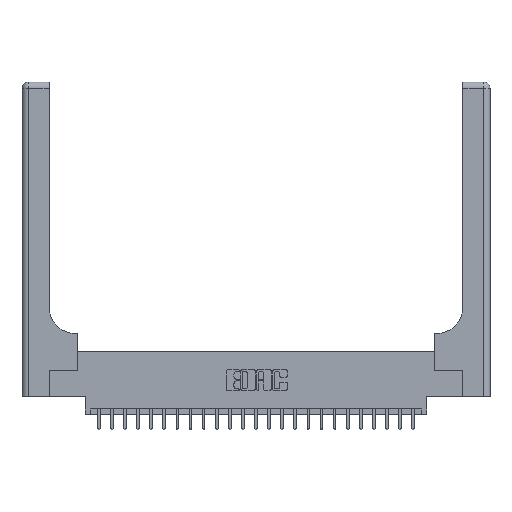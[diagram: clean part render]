
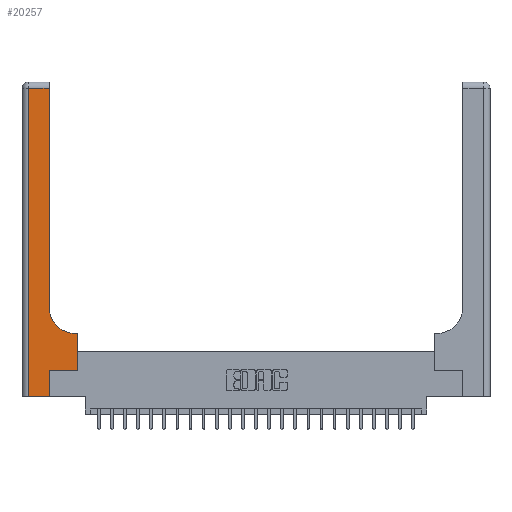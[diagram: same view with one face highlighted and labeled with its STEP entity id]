
A CAD part, top view. The second image highlights one B-rep face of the part: STEP entity #20257.
In plain terms, the highlighted planar face has unit normal (0, 0, 1).
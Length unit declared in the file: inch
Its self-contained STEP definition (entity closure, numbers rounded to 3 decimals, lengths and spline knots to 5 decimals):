
#1198 = CARTESIAN_POINT ( 'NONE',  ( 0.06, 3., 0.37 ) ) ;
#1529 = ORIENTED_EDGE ( 'NONE', *, *, #15188, .T. ) ;
#1655 = EDGE_CURVE ( 'NONE', #21835, #8231, #21204, .T. ) ;
#2003 = ORIENTED_EDGE ( 'NONE', *, *, #1655, .T. ) ;
#2154 = DIRECTION ( 'NONE',  ( 0., 1., 0. ) ) ;
#2416 = CARTESIAN_POINT ( 'NONE',  ( 0.26, 0.6, 0.37 ) ) ;
#2769 = ORIENTED_EDGE ( 'NONE', *, *, #5787, .T. ) ;
#2866 = DIRECTION ( 'NONE',  ( 1., 0., 0. ) ) ;
#3579 = DIRECTION ( 'NONE',  ( -1., 0., 0. ) ) ;
#4406 = DIRECTION ( 'NONE',  ( -1., 0., 0. ) ) ;
#4683 = DIRECTION ( 'NONE',  ( 0., 1., 0. ) ) ;
#4756 = LINE ( 'NONE', #6605, #23250 ) ;
#5188 = EDGE_CURVE ( 'NONE', #18639, #13208, #23554, .T. ) ;
#5787 = EDGE_CURVE ( 'NONE', #13319, #10318, #20450, .T. ) ;
#5858 = VERTEX_POINT ( 'NONE', #20570 ) ;
#6161 = LINE ( 'NONE', #14044, #10819 ) ;
#6267 = CARTESIAN_POINT ( 'NONE',  ( 0., 3., 0.37 ) ) ;
#6526 = ORIENTED_EDGE ( 'NONE', *, *, #8241, .T. ) ;
#6605 = CARTESIAN_POINT ( 'NONE',  ( 0.265, 0.25, 0.37 ) ) ;
#6738 = EDGE_CURVE ( 'NONE', #8231, #14518, #20949, .T. ) ;
#8231 = VERTEX_POINT ( 'NONE', #15338 ) ;
#8241 = EDGE_CURVE ( 'NONE', #13208, #13319, #6161, .T. ) ;
#8247 = DIRECTION ( 'NONE',  ( 1., 0., 0. ) ) ;
#8260 = EDGE_CURVE ( 'NONE', #5858, #18092, #11846, .T. ) ;
#8460 = VECTOR ( 'NONE', #4683, 39.37008 ) ;
#9105 = CARTESIAN_POINT ( 'NONE',  ( 0.06, 0., 0.37 ) ) ;
#9468 = CARTESIAN_POINT ( 'NONE',  ( 0.51, 0.6, 0.37 ) ) ;
#9710 = CARTESIAN_POINT ( 'NONE',  ( 0.265, 0., 0.37 ) ) ;
#9913 = EDGE_CURVE ( 'NONE', #18092, #21835, #10314, .T. ) ;
#10186 = AXIS2_PLACEMENT_3D ( 'NONE', #6267, #23171, #13796 ) ;
#10314 = LINE ( 'NONE', #2416, #19960 ) ;
#10318 = VERTEX_POINT ( 'NONE', #14209 ) ;
#10442 = VECTOR ( 'NONE', #3579, 39.37008 ) ;
#10819 = VECTOR ( 'NONE', #8247, 39.37008 ) ;
#11393 = VECTOR ( 'NONE', #19492, 39.37008 ) ;
#11846 = LINE ( 'NONE', #15560, #8460 ) ;
#13176 = CARTESIAN_POINT ( 'NONE',  ( 0.265, 0., 0.37 ) ) ;
#13208 = VERTEX_POINT ( 'NONE', #9105 ) ;
#13319 = VERTEX_POINT ( 'NONE', #9710 ) ;
#13342 = ORIENTED_EDGE ( 'NONE', *, *, #9913, .T. ) ;
#13569 = FACE_OUTER_BOUND ( 'NONE', #17978, .T. ) ;
#13658 = CARTESIAN_POINT ( 'NONE',  ( 0.26, 3., 0.37 ) ) ;
#13796 = DIRECTION ( 'NONE',  ( -1., 0., 0. ) ) ;
#14016 = CARTESIAN_POINT ( 'NONE',  ( 0.528, 0.6, 0.37 ) ) ;
#14044 = CARTESIAN_POINT ( 'NONE',  ( 0., 0., 0.37 ) ) ;
#14209 = CARTESIAN_POINT ( 'NONE',  ( 0.265, 0.25, 0.37 ) ) ;
#14497 = CARTESIAN_POINT ( 'NONE',  ( 0.06, 2.94, 0.37 ) ) ;
#14518 = VERTEX_POINT ( 'NONE', #16412 ) ;
#14719 = DIRECTION ( 'NONE',  ( 0., 0., -1. ) ) ;
#14758 = ORIENTED_EDGE ( 'NONE', *, *, #5188, .T. ) ;
#14960 = LINE ( 'NONE', #18528, #10442 ) ;
#15188 = EDGE_CURVE ( 'NONE', #14518, #18639, #14960, .T. ) ;
#15338 = CARTESIAN_POINT ( 'NONE',  ( 0.26, 0.85, 0.37 ) ) ;
#15528 = DIRECTION ( 'NONE',  ( 0., 1., 0. ) ) ;
#15560 = CARTESIAN_POINT ( 'NONE',  ( 0.528, 0.25, 0.37 ) ) ;
#15583 = VECTOR ( 'NONE', #2154, 39.37008 ) ;
#15668 = PLANE ( 'NONE',  #10186 ) ;
#16412 = CARTESIAN_POINT ( 'NONE',  ( 0.26, 2.94, 0.37 ) ) ;
#16710 = DIRECTION ( 'NONE',  ( 1., 0., 0. ) ) ;
#16916 = AXIS2_PLACEMENT_3D ( 'NONE', #22607, #14719, #16710 ) ;
#17790 = ORIENTED_EDGE ( 'NONE', *, *, #8260, .T. ) ;
#17978 = EDGE_LOOP ( 'NONE', ( #18374, #1529, #14758, #6526, #2769, #18273, #17790, #13342, #2003 ) ) ;
#18092 = VERTEX_POINT ( 'NONE', #14016 ) ;
#18273 = ORIENTED_EDGE ( 'NONE', *, *, #22832, .T. ) ;
#18374 = ORIENTED_EDGE ( 'NONE', *, *, #6738, .T. ) ;
#18528 = CARTESIAN_POINT ( 'NONE',  ( 0., 2.94, 0.37 ) ) ;
#18639 = VERTEX_POINT ( 'NONE', #14497 ) ;
#19492 = DIRECTION ( 'NONE',  ( 0., -1., 0. ) ) ;
#19960 = VECTOR ( 'NONE', #4406, 39.37008 ) ;
#20257 = ADVANCED_FACE ( 'NONE', ( #13569 ), #15668, .F. ) ;
#20450 = LINE ( 'NONE', #13176, #15583 ) ;
#20570 = CARTESIAN_POINT ( 'NONE',  ( 0.528, 0.25, 0.37 ) ) ;
#20949 = LINE ( 'NONE', #13658, #21633 ) ;
#21204 = CIRCLE ( 'NONE', #16916, 0.25 ) ;
#21633 = VECTOR ( 'NONE', #15528, 39.37008 ) ;
#21835 = VERTEX_POINT ( 'NONE', #9468 ) ;
#22607 = CARTESIAN_POINT ( 'NONE',  ( 0.51, 0.85, 0.37 ) ) ;
#22832 = EDGE_CURVE ( 'NONE', #10318, #5858, #4756, .T. ) ;
#23171 = DIRECTION ( 'NONE',  ( 0., 0., -1. ) ) ;
#23250 = VECTOR ( 'NONE', #2866, 39.37008 ) ;
#23554 = LINE ( 'NONE', #1198, #11393 ) ;
